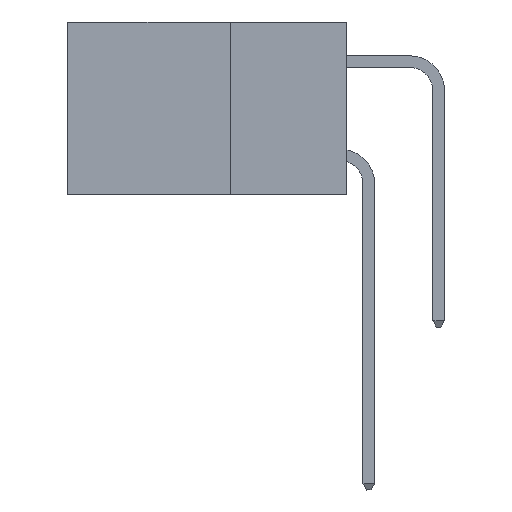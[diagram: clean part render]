
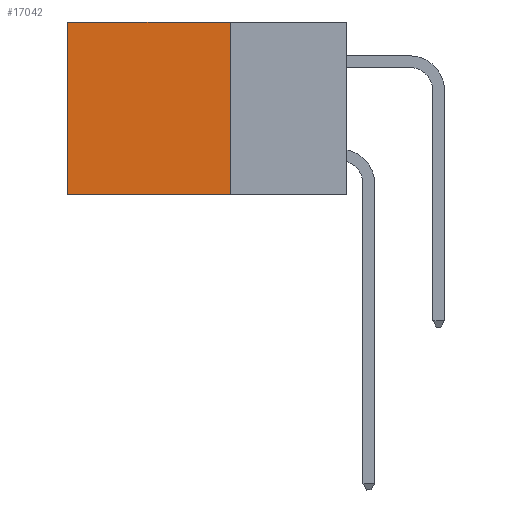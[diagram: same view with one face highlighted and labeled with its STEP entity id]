
A CAD part, left-side view. The second image highlights one B-rep face of the part: STEP entity #17042.
In plain terms, the highlighted planar face has unit normal (-1, 0, 0).
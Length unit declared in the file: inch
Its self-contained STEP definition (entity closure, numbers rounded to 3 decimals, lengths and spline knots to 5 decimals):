
#718 = LINE ( 'NONE', #13218, #2358 ) ;
#1226 = EDGE_CURVE ( 'NONE', #8123, #22614, #718, .T. ) ;
#2172 = VECTOR ( 'NONE', #6084, 39.37008 ) ;
#2358 = VECTOR ( 'NONE', #15157, 39.37008 ) ;
#4138 = ORIENTED_EDGE ( 'NONE', *, *, #14755, .T. ) ;
#4209 = DIRECTION ( 'NONE',  ( 0., 0., -1. ) ) ;
#5738 = VERTEX_POINT ( 'NONE', #8620 ) ;
#5862 = CARTESIAN_POINT ( 'NONE',  ( 0.2875, 0.25, 0. ) ) ;
#6084 = DIRECTION ( 'NONE',  ( 0., 1., 0. ) ) ;
#6100 = CARTESIAN_POINT ( 'NONE',  ( 0.2875, 0.6, 0. ) ) ;
#6159 = CARTESIAN_POINT ( 'NONE',  ( 0.2875, 0.25, -0.37 ) ) ;
#6828 = DIRECTION ( 'NONE',  ( 0., 1., 0. ) ) ;
#6854 = EDGE_CURVE ( 'NONE', #22614, #18874, #19797, .T. ) ;
#6899 = LINE ( 'NONE', #10198, #16030 ) ;
#7546 = ORIENTED_EDGE ( 'NONE', *, *, #1226, .F. ) ;
#8123 = VERTEX_POINT ( 'NONE', #5862 ) ;
#8620 = CARTESIAN_POINT ( 'NONE',  ( 0.2875, 0.6, 0. ) ) ;
#9563 = EDGE_LOOP ( 'NONE', ( #17557, #21369, #7546, #4138 ) ) ;
#9963 = CARTESIAN_POINT ( 'NONE',  ( 0.2875, 0.6, -0.37 ) ) ;
#10198 = CARTESIAN_POINT ( 'NONE',  ( 0.2875, 0.25, 0. ) ) ;
#10773 = CARTESIAN_POINT ( 'NONE',  ( 0.2875, 0.25, 0. ) ) ;
#10935 = DIRECTION ( 'NONE',  ( 1., 0., 0. ) ) ;
#12501 = CARTESIAN_POINT ( 'NONE',  ( 0.2875, 0.25, -0.37 ) ) ;
#13218 = CARTESIAN_POINT ( 'NONE',  ( 0.2875, 0.25, 0. ) ) ;
#14755 = EDGE_CURVE ( 'NONE', #8123, #5738, #6899, .T. ) ;
#15157 = DIRECTION ( 'NONE',  ( 0., 0., -1. ) ) ;
#15808 = EDGE_CURVE ( 'NONE', #5738, #18874, #19005, .T. ) ;
#16030 = VECTOR ( 'NONE', #6828, 39.37008 ) ;
#16079 = DIRECTION ( 'NONE',  ( 0., 0., -1. ) ) ;
#17042 = ADVANCED_FACE ( 'NONE', ( #18662 ), #21406, .F. ) ;
#17557 = ORIENTED_EDGE ( 'NONE', *, *, #15808, .T. ) ;
#18452 = VECTOR ( 'NONE', #4209, 39.37008 ) ;
#18662 = FACE_OUTER_BOUND ( 'NONE', #9563, .T. ) ;
#18874 = VERTEX_POINT ( 'NONE', #9963 ) ;
#19005 = LINE ( 'NONE', #6100, #18452 ) ;
#19797 = LINE ( 'NONE', #6159, #2172 ) ;
#19894 = AXIS2_PLACEMENT_3D ( 'NONE', #10773, #10935, #16079 ) ;
#21369 = ORIENTED_EDGE ( 'NONE', *, *, #6854, .F. ) ;
#21406 = PLANE ( 'NONE',  #19894 ) ;
#22614 = VERTEX_POINT ( 'NONE', #12501 ) ;
